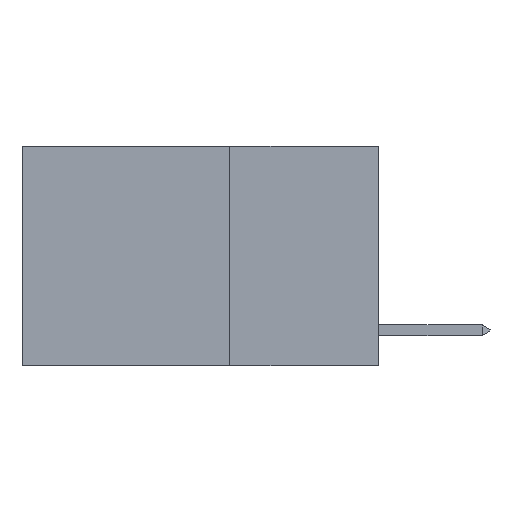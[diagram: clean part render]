
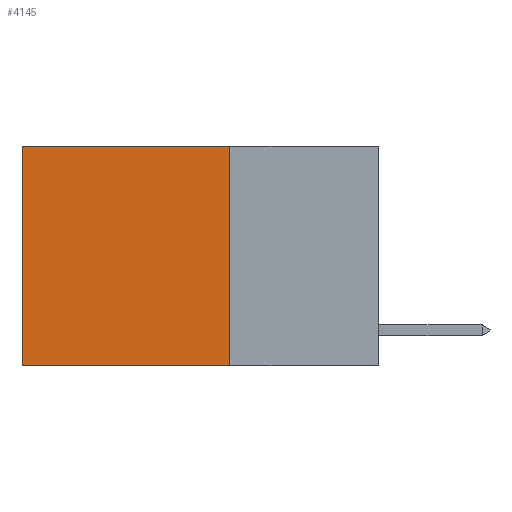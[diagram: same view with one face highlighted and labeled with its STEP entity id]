
A CAD part, left-side view. The second image highlights one B-rep face of the part: STEP entity #4145.
In plain terms, the highlighted planar face has unit normal (-1, 0, 0).
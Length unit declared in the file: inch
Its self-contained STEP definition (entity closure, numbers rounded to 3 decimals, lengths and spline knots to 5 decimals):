
#1158 = DIRECTION ( 'NONE',  ( 0., 1., 0. ) ) ;
#2276 = DIRECTION ( 'NONE',  ( 0., 0., -1. ) ) ;
#2476 = DIRECTION ( 'NONE',  ( 0., 1., 0. ) ) ;
#3311 = CARTESIAN_POINT ( 'NONE',  ( 0.2625, 0.6, 0. ) ) ;
#4145 = ADVANCED_FACE ( 'NONE', ( #21744 ), #11713, .F. ) ;
#4226 = AXIS2_PLACEMENT_3D ( 'NONE', #11801, #19101, #2276 ) ;
#4266 = LINE ( 'NONE', #21771, #14952 ) ;
#6577 = EDGE_CURVE ( 'NONE', #18219, #7011, #14645, .T. ) ;
#6658 = CARTESIAN_POINT ( 'NONE',  ( 0.2625, 0.25, -0.37 ) ) ;
#6962 = EDGE_CURVE ( 'NONE', #23868, #7011, #9282, .T. ) ;
#7011 = VERTEX_POINT ( 'NONE', #11671 ) ;
#7554 = VECTOR ( 'NONE', #2476, 39.37008 ) ;
#7578 = VECTOR ( 'NONE', #10811, 39.37008 ) ;
#7943 = EDGE_CURVE ( 'NONE', #11967, #23868, #18864, .T. ) ;
#9282 = LINE ( 'NONE', #13718, #7554 ) ;
#10021 = VECTOR ( 'NONE', #17866, 39.37008 ) ;
#10792 = CARTESIAN_POINT ( 'NONE',  ( 0.2625, 0.6, 0. ) ) ;
#10811 = DIRECTION ( 'NONE',  ( 0., 0., -1. ) ) ;
#11671 = CARTESIAN_POINT ( 'NONE',  ( 0.2625, 0.6, -0.37 ) ) ;
#11713 = PLANE ( 'NONE',  #4226 ) ;
#11801 = CARTESIAN_POINT ( 'NONE',  ( 0.2625, 0.25, 0. ) ) ;
#11967 = VERTEX_POINT ( 'NONE', #12736 ) ;
#12736 = CARTESIAN_POINT ( 'NONE',  ( 0.2625, 0.25, 0. ) ) ;
#13213 = ORIENTED_EDGE ( 'NONE', *, *, #6962, .F. ) ;
#13718 = CARTESIAN_POINT ( 'NONE',  ( 0.2625, 0.25, -0.37 ) ) ;
#14645 = LINE ( 'NONE', #3311, #10021 ) ;
#14952 = VECTOR ( 'NONE', #1158, 39.37008 ) ;
#15930 = EDGE_CURVE ( 'NONE', #11967, #18219, #4266, .T. ) ;
#17866 = DIRECTION ( 'NONE',  ( 0., 0., -1. ) ) ;
#18219 = VERTEX_POINT ( 'NONE', #10792 ) ;
#18864 = LINE ( 'NONE', #23781, #7578 ) ;
#19101 = DIRECTION ( 'NONE',  ( 1., 0., 0. ) ) ;
#20126 = EDGE_LOOP ( 'NONE', ( #21932, #13213, #21359, #21795 ) ) ;
#21359 = ORIENTED_EDGE ( 'NONE', *, *, #7943, .F. ) ;
#21744 = FACE_OUTER_BOUND ( 'NONE', #20126, .T. ) ;
#21771 = CARTESIAN_POINT ( 'NONE',  ( 0.2625, 0.25, 0. ) ) ;
#21795 = ORIENTED_EDGE ( 'NONE', *, *, #15930, .T. ) ;
#21932 = ORIENTED_EDGE ( 'NONE', *, *, #6577, .T. ) ;
#23781 = CARTESIAN_POINT ( 'NONE',  ( 0.2625, 0.25, 0. ) ) ;
#23868 = VERTEX_POINT ( 'NONE', #6658 ) ;
